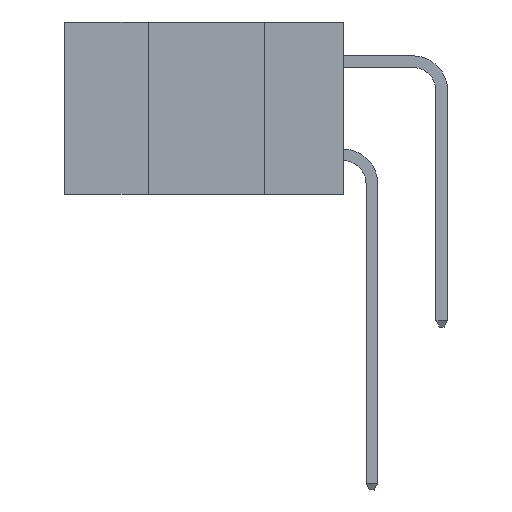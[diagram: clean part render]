
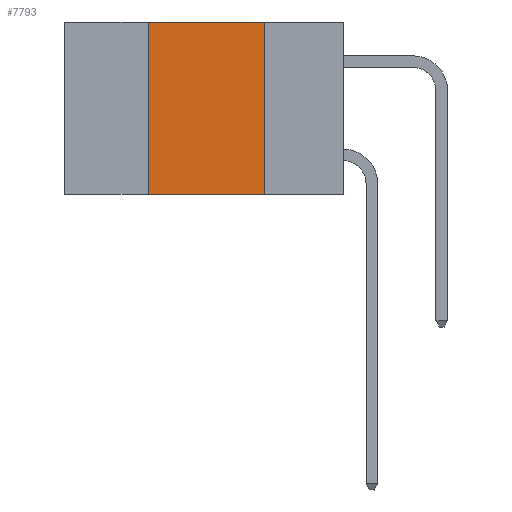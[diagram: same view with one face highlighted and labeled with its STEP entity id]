
A CAD part, left-side view. The second image highlights one B-rep face of the part: STEP entity #7793.
In plain terms, the highlighted planar face has unit normal (-1, 0, 0).
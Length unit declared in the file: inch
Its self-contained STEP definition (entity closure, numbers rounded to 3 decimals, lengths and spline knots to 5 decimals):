
#15 = CARTESIAN_POINT ( 'NONE',  ( 0., 0.42, -0.37 ) ) ;
#707 = DIRECTION ( 'NONE',  ( 0., 0., 1. ) ) ;
#1160 = CARTESIAN_POINT ( 'NONE',  ( 0., 0.42, 0. ) ) ;
#1204 = ORIENTED_EDGE ( 'NONE', *, *, #14860, .F. ) ;
#4265 = VERTEX_POINT ( 'NONE', #17745 ) ;
#4667 = EDGE_CURVE ( 'NONE', #14154, #11253, #13980, .T. ) ;
#4927 = VERTEX_POINT ( 'NONE', #15 ) ;
#4982 = DIRECTION ( 'NONE',  ( 0., -1., 0. ) ) ;
#5339 = VECTOR ( 'NONE', #707, 39.37008 ) ;
#5819 = EDGE_CURVE ( 'NONE', #4927, #4265, #9074, .T. ) ;
#5961 = CARTESIAN_POINT ( 'NONE',  ( 0., 0.6, 0. ) ) ;
#6472 = VECTOR ( 'NONE', #14562, 39.37008 ) ;
#7573 = DIRECTION ( 'NONE',  ( 1., 0., 0. ) ) ;
#7793 = ADVANCED_FACE ( 'NONE', ( #14788 ), #16060, .F. ) ;
#7987 = ORIENTED_EDGE ( 'NONE', *, *, #5819, .F. ) ;
#8340 = AXIS2_PLACEMENT_3D ( 'NONE', #14605, #7573, #17481 ) ;
#8671 = EDGE_LOOP ( 'NONE', ( #11526, #1204, #7987, #15931 ) ) ;
#9074 = LINE ( 'NONE', #1160, #5339 ) ;
#9281 = CARTESIAN_POINT ( 'NONE',  ( 0., 0.17, 0. ) ) ;
#11253 = VERTEX_POINT ( 'NONE', #13377 ) ;
#11526 = ORIENTED_EDGE ( 'NONE', *, *, #4667, .F. ) ;
#12819 = CARTESIAN_POINT ( 'NONE',  ( 0., 0.17, 0. ) ) ;
#13048 = DIRECTION ( 'NONE',  ( 0., -1., 0. ) ) ;
#13175 = EDGE_CURVE ( 'NONE', #4927, #11253, #16933, .T. ) ;
#13377 = CARTESIAN_POINT ( 'NONE',  ( 0., 0.17, -0.37 ) ) ;
#13940 = VECTOR ( 'NONE', #13048, 39.37008 ) ;
#13980 = LINE ( 'NONE', #9281, #6472 ) ;
#14154 = VERTEX_POINT ( 'NONE', #12819 ) ;
#14562 = DIRECTION ( 'NONE',  ( 0., 0., -1. ) ) ;
#14605 = CARTESIAN_POINT ( 'NONE',  ( 0., 0.6, 0. ) ) ;
#14788 = FACE_OUTER_BOUND ( 'NONE', #8671, .T. ) ;
#14851 = CARTESIAN_POINT ( 'NONE',  ( 0., 0.6, -0.37 ) ) ;
#14860 = EDGE_CURVE ( 'NONE', #4265, #14154, #17749, .T. ) ;
#15931 = ORIENTED_EDGE ( 'NONE', *, *, #13175, .T. ) ;
#16060 = PLANE ( 'NONE',  #8340 ) ;
#16933 = LINE ( 'NONE', #14851, #17824 ) ;
#17481 = DIRECTION ( 'NONE',  ( 0., 0., -1. ) ) ;
#17745 = CARTESIAN_POINT ( 'NONE',  ( 0., 0.42, 0. ) ) ;
#17749 = LINE ( 'NONE', #5961, #13940 ) ;
#17824 = VECTOR ( 'NONE', #4982, 39.37008 ) ;
